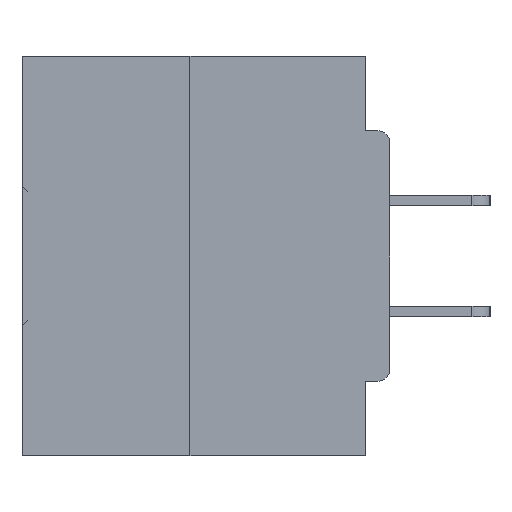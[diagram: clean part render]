
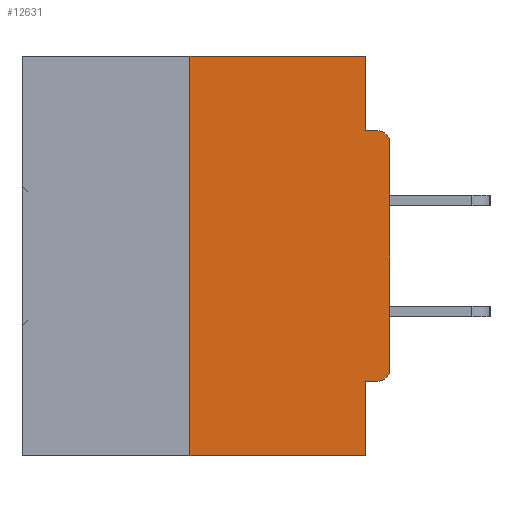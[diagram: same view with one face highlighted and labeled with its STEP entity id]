
A CAD part, left-side view. The second image highlights one B-rep face of the part: STEP entity #12631.
In plain terms, the highlighted planar face has unit normal (-1, 0, 0).
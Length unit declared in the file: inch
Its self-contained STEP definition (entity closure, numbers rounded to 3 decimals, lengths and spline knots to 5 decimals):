
#942 = EDGE_LOOP ( 'NONE', ( #32141, #17599, #21156, #39443, #36461, #35436, #29403, #39390, #17183, #15901 ) ) ;
#963 = CIRCLE ( 'NONE', #34989, 0.015 ) ;
#1891 = EDGE_CURVE ( 'NONE', #10869, #7916, #26112, .T. ) ;
#2251 = DIRECTION ( 'NONE',  ( 1., 0., 0. ) ) ;
#3830 = LINE ( 'NONE', #9960, #13963 ) ;
#5081 = VERTEX_POINT ( 'NONE', #38687 ) ;
#7649 = LINE ( 'NONE', #9907, #32879 ) ;
#7819 = EDGE_CURVE ( 'NONE', #46436, #43539, #40537, .T. ) ;
#7916 = VERTEX_POINT ( 'NONE', #43296 ) ;
#8067 = CARTESIAN_POINT ( 'NONE',  ( 0., 0.031, -0.5 ) ) ;
#8389 = FACE_OUTER_BOUND ( 'NONE', #942, .T. ) ;
#8747 = CARTESIAN_POINT ( 'NONE',  ( 0., 0.015, -0.1085 ) ) ;
#8875 = VERTEX_POINT ( 'NONE', #46495 ) ;
#9188 = CARTESIAN_POINT ( 'NONE',  ( 0., 0.46, 0. ) ) ;
#9245 = LINE ( 'NONE', #22057, #17101 ) ;
#9287 = VERTEX_POINT ( 'NONE', #31722 ) ;
#9535 = CARTESIAN_POINT ( 'NONE',  ( 0., 0.015, -0.4065 ) ) ;
#9794 = LINE ( 'NONE', #40530, #10923 ) ;
#9907 = CARTESIAN_POINT ( 'NONE',  ( 0., 0.46, -0.5 ) ) ;
#9960 = CARTESIAN_POINT ( 'NONE',  ( 0., 0., -0.0935 ) ) ;
#10869 = VERTEX_POINT ( 'NONE', #37699 ) ;
#10923 = VECTOR ( 'NONE', #22766, 39.37008 ) ;
#12300 = CARTESIAN_POINT ( 'NONE',  ( 0., 0.031, -0.0935 ) ) ;
#12631 = ADVANCED_FACE ( 'NONE', ( #8389 ), #16567, .F. ) ;
#12925 = EDGE_CURVE ( 'NONE', #17464, #8875, #3830, .T. ) ;
#13110 = DIRECTION ( 'NONE',  ( 0., 0., -1. ) ) ;
#13355 = DIRECTION ( 'NONE',  ( 0., 0., 1. ) ) ;
#13574 = CARTESIAN_POINT ( 'NONE',  ( 0., 0., 0. ) ) ;
#13963 = VECTOR ( 'NONE', #45904, 39.37008 ) ;
#14498 = CARTESIAN_POINT ( 'NONE',  ( 0., 0.25, -0.5 ) ) ;
#14604 = EDGE_CURVE ( 'NONE', #21213, #17464, #9245, .T. ) ;
#14946 = VECTOR ( 'NONE', #45916, 39.37008 ) ;
#15414 = AXIS2_PLACEMENT_3D ( 'NONE', #9188, #2251, #13110 ) ;
#15901 = ORIENTED_EDGE ( 'NONE', *, *, #14604, .F. ) ;
#15975 = CIRCLE ( 'NONE', #17685, 0.015 ) ;
#16567 = PLANE ( 'NONE',  #15414 ) ;
#17101 = VECTOR ( 'NONE', #36178, 39.37008 ) ;
#17183 = ORIENTED_EDGE ( 'NONE', *, *, #12925, .F. ) ;
#17464 = VERTEX_POINT ( 'NONE', #12300 ) ;
#17599 = ORIENTED_EDGE ( 'NONE', *, *, #7819, .F. ) ;
#17685 = AXIS2_PLACEMENT_3D ( 'NONE', #8747, #33802, #19565 ) ;
#18384 = CARTESIAN_POINT ( 'NONE',  ( 0., 0.25, 0. ) ) ;
#18400 = CARTESIAN_POINT ( 'NONE',  ( 0., 0.015, -0.3915 ) ) ;
#19565 = DIRECTION ( 'NONE',  ( 0., 0., -1. ) ) ;
#20371 = EDGE_CURVE ( 'NONE', #23800, #10869, #9794, .T. ) ;
#21156 = ORIENTED_EDGE ( 'NONE', *, *, #25470, .T. ) ;
#21213 = VERTEX_POINT ( 'NONE', #29833 ) ;
#21607 = VECTOR ( 'NONE', #29231, 39.37008 ) ;
#22057 = CARTESIAN_POINT ( 'NONE',  ( 0., 0.031, 0. ) ) ;
#22368 = EDGE_CURVE ( 'NONE', #43539, #21213, #40789, .T. ) ;
#22612 = DIRECTION ( 'NONE',  ( 0., 0., -1. ) ) ;
#22766 = DIRECTION ( 'NONE',  ( 0., 1., 0. ) ) ;
#22818 = DIRECTION ( 'NONE',  ( 0., -1., 0. ) ) ;
#23215 = CARTESIAN_POINT ( 'NONE',  ( 0., 0.25, 0. ) ) ;
#23338 = VECTOR ( 'NONE', #22818, 39.37008 ) ;
#23800 = VERTEX_POINT ( 'NONE', #9535 ) ;
#24253 = EDGE_CURVE ( 'NONE', #23800, #9287, #963, .T. ) ;
#25470 = EDGE_CURVE ( 'NONE', #46436, #7916, #7649, .T. ) ;
#26112 = LINE ( 'NONE', #8067, #21607 ) ;
#26455 = VECTOR ( 'NONE', #13355, 39.37008 ) ;
#26728 = CARTESIAN_POINT ( 'NONE',  ( 0., 0.46, 0. ) ) ;
#28900 = EDGE_CURVE ( 'NONE', #5081, #8875, #15975, .T. ) ;
#29231 = DIRECTION ( 'NONE',  ( 0., 0., -1. ) ) ;
#29403 = ORIENTED_EDGE ( 'NONE', *, *, #34283, .T. ) ;
#29833 = CARTESIAN_POINT ( 'NONE',  ( 0., 0.031, 0. ) ) ;
#31242 = LINE ( 'NONE', #13574, #14946 ) ;
#31722 = CARTESIAN_POINT ( 'NONE',  ( 0., 0., -0.3915 ) ) ;
#32141 = ORIENTED_EDGE ( 'NONE', *, *, #22368, .F. ) ;
#32879 = VECTOR ( 'NONE', #45545, 39.37008 ) ;
#33802 = DIRECTION ( 'NONE',  ( -1., 0., 0. ) ) ;
#34283 = EDGE_CURVE ( 'NONE', #9287, #5081, #31242, .T. ) ;
#34989 = AXIS2_PLACEMENT_3D ( 'NONE', #18400, #43529, #22612 ) ;
#35436 = ORIENTED_EDGE ( 'NONE', *, *, #24253, .T. ) ;
#36178 = DIRECTION ( 'NONE',  ( 0., 0., -1. ) ) ;
#36461 = ORIENTED_EDGE ( 'NONE', *, *, #20371, .F. ) ;
#37699 = CARTESIAN_POINT ( 'NONE',  ( 0., 0.031, -0.4065 ) ) ;
#38687 = CARTESIAN_POINT ( 'NONE',  ( 0., 0., -0.1085 ) ) ;
#39390 = ORIENTED_EDGE ( 'NONE', *, *, #28900, .T. ) ;
#39443 = ORIENTED_EDGE ( 'NONE', *, *, #1891, .F. ) ;
#40530 = CARTESIAN_POINT ( 'NONE',  ( 0., 0., -0.4065 ) ) ;
#40537 = LINE ( 'NONE', #23215, #26455 ) ;
#40789 = LINE ( 'NONE', #26728, #23338 ) ;
#43296 = CARTESIAN_POINT ( 'NONE',  ( 0., 0.031, -0.5 ) ) ;
#43529 = DIRECTION ( 'NONE',  ( -1., 0., 0. ) ) ;
#43539 = VERTEX_POINT ( 'NONE', #18384 ) ;
#45545 = DIRECTION ( 'NONE',  ( 0., -1., 0. ) ) ;
#45904 = DIRECTION ( 'NONE',  ( 0., -1., 0. ) ) ;
#45916 = DIRECTION ( 'NONE',  ( 0., 0., 1. ) ) ;
#46436 = VERTEX_POINT ( 'NONE', #14498 ) ;
#46495 = CARTESIAN_POINT ( 'NONE',  ( 0., 0.015, -0.0935 ) ) ;
